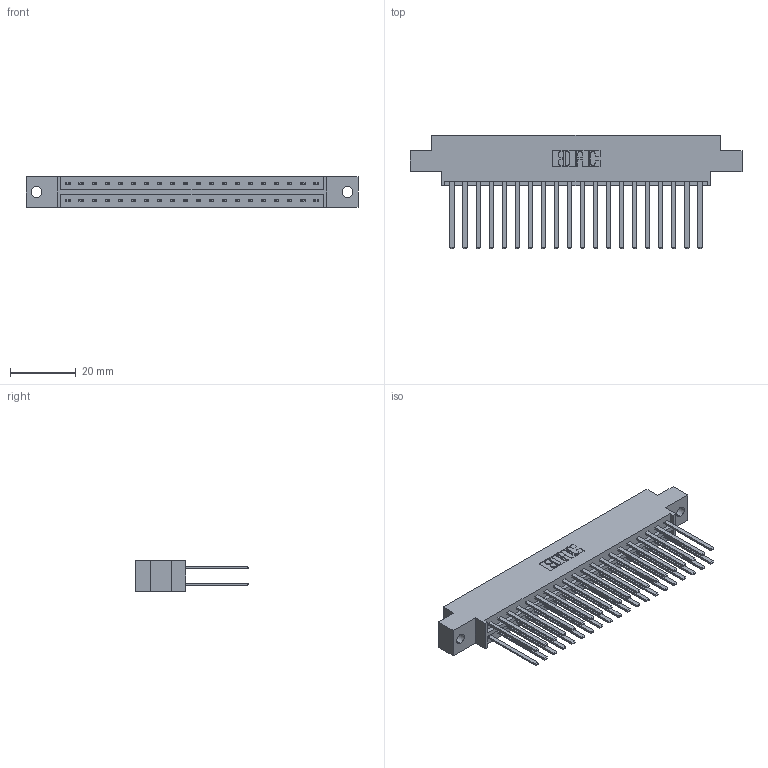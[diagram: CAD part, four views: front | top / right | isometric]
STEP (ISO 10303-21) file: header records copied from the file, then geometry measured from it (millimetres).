
FILE_DESCRIPTION (( 'STEP AP203' ), '1' );
FILE_NAME ('833-040-544-802.STEP', '2020-06-03T17:34:38', ( '' ), ( '' ), 'SwSTEP 2.0', 'SolidWorks 2020', '' );
FILE_SCHEMA (( 'CONFIG_CONTROL_DESIGN' ));
Length unit declared in the file: inch
Products named in the file (3): 345-292-001_345-293-144; 833 Part_Offset - .128 Dia; 833-040-544-802
Assembly tree (41 placements, depth 2):
  833-040-544-802
    833 Part_Offset - .128 Dia
    345-292-001_345-293-144  x40
Bounding box: 100.79 x 34.3 x 9.4 mm (x, y, z)
Volume: 10380.3 mm3; surface area: 13788.6 mm2
Topology: 41 solids, 41 shells, 1958 faces, 5803 edges, 3814 vertices
Faces by surface type: plane 1354, cylinder 604
Entity records: 15663 total; most frequent: CARTESIAN_POINT 2622, ORIENTED_EDGE 2558, DIRECTION 2275, EDGE_CURVE 1279, VECTOR 1155, LINE 1155, VERTEX_POINT 850, AXIS2_PLACEMENT_3D 560
